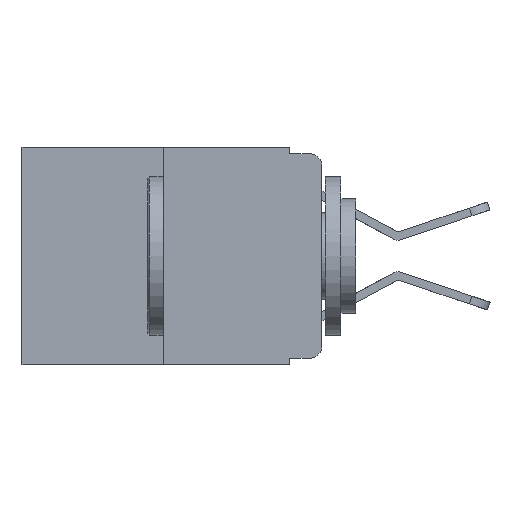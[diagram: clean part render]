
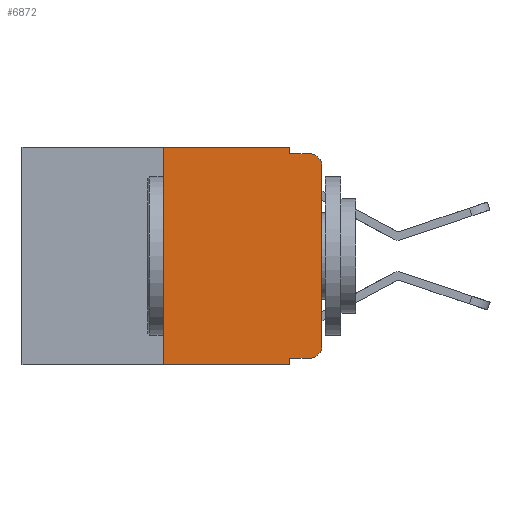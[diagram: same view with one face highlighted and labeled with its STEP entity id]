
A CAD part, left-side view. The second image highlights one B-rep face of the part: STEP entity #6872.
In plain terms, the highlighted planar face has unit normal (-1, 0, 0).
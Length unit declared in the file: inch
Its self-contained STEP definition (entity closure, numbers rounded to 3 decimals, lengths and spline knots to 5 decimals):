
#93 = CARTESIAN_POINT ( 'NONE',  ( 0., 0.051, -0.333 ) ) ;
#607 = VERTEX_POINT ( 'NONE', #5967 ) ;
#840 = DIRECTION ( 'NONE',  ( 0., -1., 0. ) ) ;
#969 = VECTOR ( 'NONE', #5364, 39.37008 ) ;
#1034 = VERTEX_POINT ( 'NONE', #8816 ) ;
#1126 = CARTESIAN_POINT ( 'NONE',  ( 0., 0.051, -0.343 ) ) ;
#1456 = DIRECTION ( 'NONE',  ( -1., 0., 0. ) ) ;
#2129 = CARTESIAN_POINT ( 'NONE',  ( 0., 0.473, -0.343 ) ) ;
#2179 = CARTESIAN_POINT ( 'NONE',  ( 0., 0.051, 0. ) ) ;
#2846 = DIRECTION ( 'NONE',  ( 0., 0., -1. ) ) ;
#2964 = VECTOR ( 'NONE', #7796, 39.37008 ) ;
#3125 = LINE ( 'NONE', #8742, #9287 ) ;
#3187 = DIRECTION ( 'NONE',  ( 0., 0., -1. ) ) ;
#3369 = CARTESIAN_POINT ( 'NONE',  ( 0., 0., -0.313 ) ) ;
#3459 = ORIENTED_EDGE ( 'NONE', *, *, #6377, .F. ) ;
#3561 = EDGE_CURVE ( 'NONE', #14301, #607, #5372, .T. ) ;
#3785 = LINE ( 'NONE', #9429, #8781 ) ;
#3818 = VERTEX_POINT ( 'NONE', #3369 ) ;
#3903 = VERTEX_POINT ( 'NONE', #12435 ) ;
#3914 = CARTESIAN_POINT ( 'NONE',  ( 0., 0., 0. ) ) ;
#4430 = VERTEX_POINT ( 'NONE', #1126 ) ;
#4752 = CARTESIAN_POINT ( 'NONE',  ( 0., 0.473, 0. ) ) ;
#5276 = EDGE_CURVE ( 'NONE', #3818, #14301, #15208, .T. ) ;
#5347 = CARTESIAN_POINT ( 'NONE',  ( 0., 0.473, 0. ) ) ;
#5364 = DIRECTION ( 'NONE',  ( 0., 0., 1. ) ) ;
#5372 = CIRCLE ( 'NONE', #7740, 0.02 ) ;
#5595 = ORIENTED_EDGE ( 'NONE', *, *, #8465, .F. ) ;
#5731 = DIRECTION ( 'NONE',  ( 0., -1., 0. ) ) ;
#5967 = CARTESIAN_POINT ( 'NONE',  ( 0., 0.02, -0.01 ) ) ;
#6017 = CIRCLE ( 'NONE', #15786, 0.02 ) ;
#6244 = VECTOR ( 'NONE', #840, 39.37008 ) ;
#6347 = VERTEX_POINT ( 'NONE', #13395 ) ;
#6377 = EDGE_CURVE ( 'NONE', #9044, #4430, #11130, .T. ) ;
#6416 = LINE ( 'NONE', #4752, #13549 ) ;
#6872 = ADVANCED_FACE ( 'NONE', ( #17965 ), #9543, .F. ) ;
#7056 = EDGE_CURVE ( 'NONE', #9044, #1034, #7106, .T. ) ;
#7106 = LINE ( 'NONE', #93, #13583 ) ;
#7236 = DIRECTION ( 'NONE',  ( -1., 0., 0. ) ) ;
#7340 = DIRECTION ( 'NONE',  ( 0., 0., 1. ) ) ;
#7387 = ORIENTED_EDGE ( 'NONE', *, *, #7056, .T. ) ;
#7405 = CARTESIAN_POINT ( 'NONE',  ( 0., 0.02, -0.03 ) ) ;
#7740 = AXIS2_PLACEMENT_3D ( 'NONE', #7405, #7236, #3187 ) ;
#7796 = DIRECTION ( 'NONE',  ( 0., 0., -1. ) ) ;
#8238 = CARTESIAN_POINT ( 'NONE',  ( 0., 0.051, 0. ) ) ;
#8465 = EDGE_CURVE ( 'NONE', #9817, #607, #3785, .T. ) ;
#8737 = CARTESIAN_POINT ( 'NONE',  ( 0., 0.051, -0.333 ) ) ;
#8742 = CARTESIAN_POINT ( 'NONE',  ( 0., 0.25, 0. ) ) ;
#8781 = VECTOR ( 'NONE', #15079, 39.37008 ) ;
#8784 = EDGE_LOOP ( 'NONE', ( #12777, #17043, #5595, #16083, #17130, #13763, #13526, #3459, #7387, #15131 ) ) ;
#8816 = CARTESIAN_POINT ( 'NONE',  ( 0., 0.02, -0.333 ) ) ;
#9044 = VERTEX_POINT ( 'NONE', #8737 ) ;
#9200 = LINE ( 'NONE', #2179, #2964 ) ;
#9218 = EDGE_CURVE ( 'NONE', #6347, #3903, #6416, .T. ) ;
#9287 = VECTOR ( 'NONE', #7340, 39.37008 ) ;
#9429 = CARTESIAN_POINT ( 'NONE',  ( 0., 0.051, -0.01 ) ) ;
#9543 = PLANE ( 'NONE',  #17290 ) ;
#9638 = DIRECTION ( 'NONE',  ( 1., 0., 0. ) ) ;
#9817 = VERTEX_POINT ( 'NONE', #11430 ) ;
#10050 = CARTESIAN_POINT ( 'NONE',  ( 0., 0.02, -0.313 ) ) ;
#10691 = DIRECTION ( 'NONE',  ( 0., 0., -1. ) ) ;
#10794 = VECTOR ( 'NONE', #10691, 39.37008 ) ;
#11130 = LINE ( 'NONE', #8238, #10794 ) ;
#11430 = CARTESIAN_POINT ( 'NONE',  ( 0., 0.051, -0.01 ) ) ;
#11889 = DIRECTION ( 'NONE',  ( 0., -1., 0. ) ) ;
#12435 = CARTESIAN_POINT ( 'NONE',  ( 0., 0.051, 0. ) ) ;
#12608 = EDGE_CURVE ( 'NONE', #3903, #9817, #9200, .T. ) ;
#12777 = ORIENTED_EDGE ( 'NONE', *, *, #5276, .T. ) ;
#13395 = CARTESIAN_POINT ( 'NONE',  ( 0., 0.25, 0. ) ) ;
#13526 = ORIENTED_EDGE ( 'NONE', *, *, #14539, .T. ) ;
#13549 = VECTOR ( 'NONE', #11889, 39.37008 ) ;
#13583 = VECTOR ( 'NONE', #5731, 39.37008 ) ;
#13763 = ORIENTED_EDGE ( 'NONE', *, *, #16597, .F. ) ;
#14301 = VERTEX_POINT ( 'NONE', #15395 ) ;
#14459 = VERTEX_POINT ( 'NONE', #14546 ) ;
#14539 = EDGE_CURVE ( 'NONE', #14459, #4430, #17390, .T. ) ;
#14546 = CARTESIAN_POINT ( 'NONE',  ( 0., 0.25, -0.343 ) ) ;
#15079 = DIRECTION ( 'NONE',  ( 0., -1., 0. ) ) ;
#15131 = ORIENTED_EDGE ( 'NONE', *, *, #18132, .T. ) ;
#15208 = LINE ( 'NONE', #3914, #969 ) ;
#15395 = CARTESIAN_POINT ( 'NONE',  ( 0., 0., -0.03 ) ) ;
#15786 = AXIS2_PLACEMENT_3D ( 'NONE', #10050, #1456, #2846 ) ;
#16083 = ORIENTED_EDGE ( 'NONE', *, *, #12608, .F. ) ;
#16597 = EDGE_CURVE ( 'NONE', #14459, #6347, #3125, .T. ) ;
#16675 = DIRECTION ( 'NONE',  ( 0., 0., -1. ) ) ;
#17043 = ORIENTED_EDGE ( 'NONE', *, *, #3561, .T. ) ;
#17130 = ORIENTED_EDGE ( 'NONE', *, *, #9218, .F. ) ;
#17290 = AXIS2_PLACEMENT_3D ( 'NONE', #5347, #9638, #16675 ) ;
#17390 = LINE ( 'NONE', #2129, #6244 ) ;
#17965 = FACE_OUTER_BOUND ( 'NONE', #8784, .T. ) ;
#18132 = EDGE_CURVE ( 'NONE', #1034, #3818, #6017, .T. ) ;
